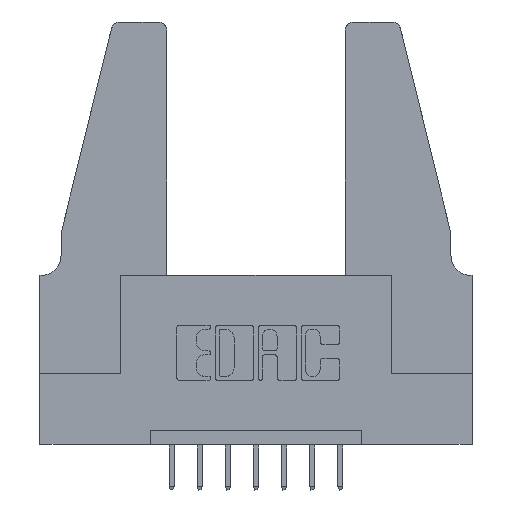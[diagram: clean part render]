
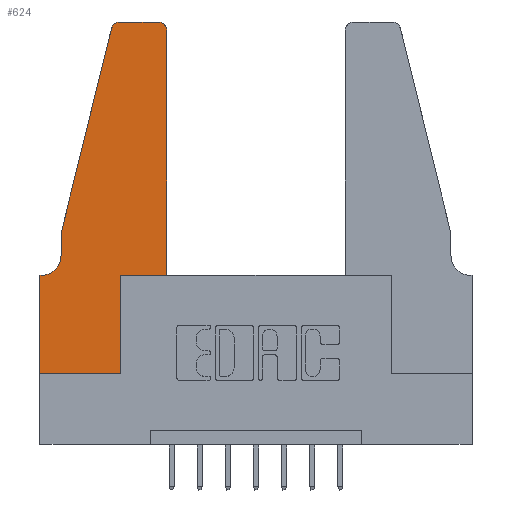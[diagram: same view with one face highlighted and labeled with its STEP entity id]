
A CAD part, top view. The second image highlights one B-rep face of the part: STEP entity #624.
In plain terms, the highlighted planar face has unit normal (0, 0, 1).
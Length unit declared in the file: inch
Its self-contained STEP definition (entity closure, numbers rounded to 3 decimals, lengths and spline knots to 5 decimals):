
#6 = VECTOR ( 'NONE', #4081, 39.37008 ) ;
#82 = CARTESIAN_POINT ( 'NONE',  ( 0.25487, 1.22718, 0.37 ) ) ;
#151 = VERTEX_POINT ( 'NONE', #7813 ) ;
#403 = CARTESIAN_POINT ( 'NONE',  ( 0.0755, 0.35, 0.37 ) ) ;
#438 = DIRECTION ( 'NONE',  ( -1., 0., 0. ) ) ;
#596 = ORIENTED_EDGE ( 'NONE', *, *, #9258, .T. ) ;
#624 = ADVANCED_FACE ( 'NONE', ( #4586 ), #5014, .T. ) ;
#721 = CARTESIAN_POINT ( 'NONE',  ( 0., 0., 0.37 ) ) ;
#896 = DIRECTION ( 'NONE',  ( 0., 1., 0. ) ) ;
#988 = VERTEX_POINT ( 'NONE', #82 ) ;
#1193 = EDGE_CURVE ( 'NONE', #5712, #9360, #9773, .T. ) ;
#1250 = ORIENTED_EDGE ( 'NONE', *, *, #1193, .T. ) ;
#1460 = DIRECTION ( 'NONE',  ( 0., 1., 0. ) ) ;
#1491 = CARTESIAN_POINT ( 'NONE',  ( 0., 0.35, 0.37 ) ) ;
#1648 = VECTOR ( 'NONE', #3179, 39.37008 ) ;
#1734 = EDGE_CURVE ( 'NONE', #6615, #151, #4165, .T. ) ;
#1906 = LINE ( 'NONE', #8679, #4118 ) ;
#1989 = DIRECTION ( 'NONE',  ( 0., 0., 1. ) ) ;
#2083 = EDGE_CURVE ( 'NONE', #11828, #5712, #11872, .T. ) ;
#2262 = EDGE_CURVE ( 'NONE', #11315, #8627, #3026, .T. ) ;
#2263 = CARTESIAN_POINT ( 'NONE',  ( 0.4505, 0.35, 0.37 ) ) ;
#2311 = CARTESIAN_POINT ( 'NONE',  ( 0., 0.35, 0.37 ) ) ;
#2514 = CARTESIAN_POINT ( 'NONE',  ( 0.4505, 0.35, 0.37 ) ) ;
#2665 = EDGE_CURVE ( 'NONE', #8627, #6615, #6986, .T. ) ;
#2814 = DIRECTION ( 'NONE',  ( 0., 0., 1. ) ) ;
#2818 = DIRECTION ( 'NONE',  ( 0., -1., 0. ) ) ;
#2989 = EDGE_CURVE ( 'NONE', #988, #11828, #6393, .T. ) ;
#3023 = DIRECTION ( 'NONE',  ( -0.239, -0.971, 0. ) ) ;
#3026 = LINE ( 'NONE', #5079, #7000 ) ;
#3153 = CARTESIAN_POINT ( 'NONE',  ( 0.4505, 1.22, 0.37 ) ) ;
#3179 = DIRECTION ( 'NONE',  ( -1., 0., 0. ) ) ;
#3207 = EDGE_CURVE ( 'NONE', #6778, #11315, #8769, .T. ) ;
#3413 = LINE ( 'NONE', #12219, #4577 ) ;
#3459 = VECTOR ( 'NONE', #5008, 39.37008 ) ;
#3604 = EDGE_LOOP ( 'NONE', ( #10186, #596, #9419, #10595, #1250, #5527, #6109, #10179, #5342, #10433, #5573, #6442 ) ) ;
#3886 = AXIS2_PLACEMENT_3D ( 'NONE', #2311, #1989, #11776 ) ;
#3912 = DIRECTION ( 'NONE',  ( 0., 0., 1. ) ) ;
#4081 = DIRECTION ( 'NONE',  ( -1., 0., 0. ) ) ;
#4095 = CARTESIAN_POINT ( 'NONE',  ( 0.2605, 1.25, 0.37 ) ) ;
#4118 = VECTOR ( 'NONE', #11498, 39.37008 ) ;
#4165 = LINE ( 'NONE', #4095, #1648 ) ;
#4577 = VECTOR ( 'NONE', #896, 39.37008 ) ;
#4586 = FACE_OUTER_BOUND ( 'NONE', #3604, .T. ) ;
#4598 = CARTESIAN_POINT ( 'NONE',  ( 0.0755, 0.5, 0.37 ) ) ;
#4817 = CARTESIAN_POINT ( 'NONE',  ( 0.2865, 0., 0.37 ) ) ;
#4829 = EDGE_CURVE ( 'NONE', #4919, #6778, #3413, .T. ) ;
#4919 = VERTEX_POINT ( 'NONE', #4817 ) ;
#4946 = DIRECTION ( 'NONE',  ( 0., 0., -1. ) ) ;
#5008 = DIRECTION ( 'NONE',  ( 1., 0., 0. ) ) ;
#5014 = PLANE ( 'NONE',  #3886 ) ;
#5079 = CARTESIAN_POINT ( 'NONE',  ( 0.4505, 0.35, 0.37 ) ) ;
#5342 = ORIENTED_EDGE ( 'NONE', *, *, #4829, .T. ) ;
#5381 = CARTESIAN_POINT ( 'NONE',  ( 0.2865, 0.35, 0.37 ) ) ;
#5527 = ORIENTED_EDGE ( 'NONE', *, *, #6477, .T. ) ;
#5568 = DIRECTION ( 'NONE',  ( 1., 0., 0. ) ) ;
#5573 = ORIENTED_EDGE ( 'NONE', *, *, #2262, .T. ) ;
#5654 = CARTESIAN_POINT ( 'NONE',  ( 0.0055, 0.35, 0.37 ) ) ;
#5712 = VERTEX_POINT ( 'NONE', #6344 ) ;
#6109 = ORIENTED_EDGE ( 'NONE', *, *, #9649, .T. ) ;
#6344 = CARTESIAN_POINT ( 'NONE',  ( 0.0755, 0.42, 0.37 ) ) ;
#6393 = LINE ( 'NONE', #8676, #8464 ) ;
#6442 = ORIENTED_EDGE ( 'NONE', *, *, #2665, .T. ) ;
#6477 = EDGE_CURVE ( 'NONE', #9360, #7540, #9287, .T. ) ;
#6615 = VERTEX_POINT ( 'NONE', #11170 ) ;
#6778 = VERTEX_POINT ( 'NONE', #5381 ) ;
#6916 = CARTESIAN_POINT ( 'NONE',  ( 0.0755, 0.5, 0.37 ) ) ;
#6986 = CIRCLE ( 'NONE', #10159, 0.03 ) ;
#7000 = VECTOR ( 'NONE', #1460, 39.37008 ) ;
#7427 = AXIS2_PLACEMENT_3D ( 'NONE', #10646, #4946, #438 ) ;
#7540 = VERTEX_POINT ( 'NONE', #1491 ) ;
#7813 = CARTESIAN_POINT ( 'NONE',  ( 0.284, 1.25, 0.37 ) ) ;
#8062 = VECTOR ( 'NONE', #8947, 39.37008 ) ;
#8428 = EDGE_CURVE ( 'NONE', #9918, #4919, #1906, .T. ) ;
#8464 = VECTOR ( 'NONE', #3023, 39.37008 ) ;
#8604 = DIRECTION ( 'NONE',  ( 1., 0., 0. ) ) ;
#8627 = VERTEX_POINT ( 'NONE', #3153 ) ;
#8641 = CIRCLE ( 'NONE', #11431, 0.03 ) ;
#8676 = CARTESIAN_POINT ( 'NONE',  ( 0.0755, 0.5, 0.37 ) ) ;
#8679 = CARTESIAN_POINT ( 'NONE',  ( 0., 0., 0.37 ) ) ;
#8769 = LINE ( 'NONE', #2263, #3459 ) ;
#8947 = DIRECTION ( 'NONE',  ( 0., -1., 0. ) ) ;
#9258 = EDGE_CURVE ( 'NONE', #151, #988, #8641, .T. ) ;
#9287 = LINE ( 'NONE', #403, #6 ) ;
#9328 = VECTOR ( 'NONE', #2818, 39.37008 ) ;
#9360 = VERTEX_POINT ( 'NONE', #5654 ) ;
#9419 = ORIENTED_EDGE ( 'NONE', *, *, #2989, .T. ) ;
#9649 = EDGE_CURVE ( 'NONE', #7540, #9918, #11949, .T. ) ;
#9773 = CIRCLE ( 'NONE', #7427, 0.07 ) ;
#9918 = VERTEX_POINT ( 'NONE', #721 ) ;
#10159 = AXIS2_PLACEMENT_3D ( 'NONE', #10316, #2814, #5568 ) ;
#10179 = ORIENTED_EDGE ( 'NONE', *, *, #8428, .T. ) ;
#10186 = ORIENTED_EDGE ( 'NONE', *, *, #1734, .T. ) ;
#10316 = CARTESIAN_POINT ( 'NONE',  ( 0.4205, 1.22, 0.37 ) ) ;
#10433 = ORIENTED_EDGE ( 'NONE', *, *, #3207, .T. ) ;
#10437 = CARTESIAN_POINT ( 'NONE',  ( 0.284, 1.22, 0.37 ) ) ;
#10595 = ORIENTED_EDGE ( 'NONE', *, *, #2083, .T. ) ;
#10646 = CARTESIAN_POINT ( 'NONE',  ( 0.0055, 0.42, 0.37 ) ) ;
#11170 = CARTESIAN_POINT ( 'NONE',  ( 0.4205, 1.25, 0.37 ) ) ;
#11315 = VERTEX_POINT ( 'NONE', #2514 ) ;
#11431 = AXIS2_PLACEMENT_3D ( 'NONE', #10437, #3912, #8604 ) ;
#11498 = DIRECTION ( 'NONE',  ( 1., 0., 0. ) ) ;
#11776 = DIRECTION ( 'NONE',  ( 1., 0., 0. ) ) ;
#11828 = VERTEX_POINT ( 'NONE', #6916 ) ;
#11872 = LINE ( 'NONE', #4598, #9328 ) ;
#11919 = CARTESIAN_POINT ( 'NONE',  ( 0., 0., 0.37 ) ) ;
#11949 = LINE ( 'NONE', #11919, #8062 ) ;
#12219 = CARTESIAN_POINT ( 'NONE',  ( 0.2865, 0.35, 0.37 ) ) ;
